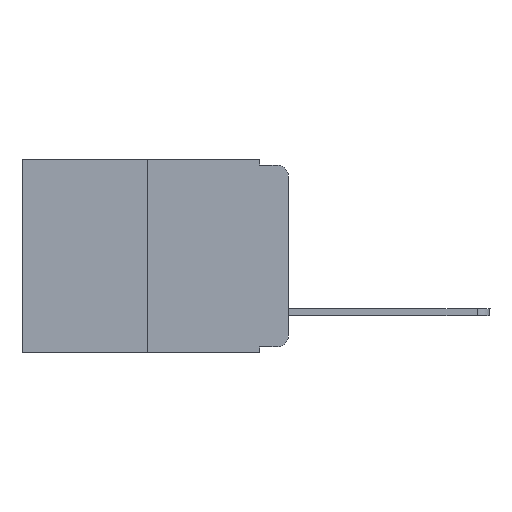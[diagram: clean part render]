
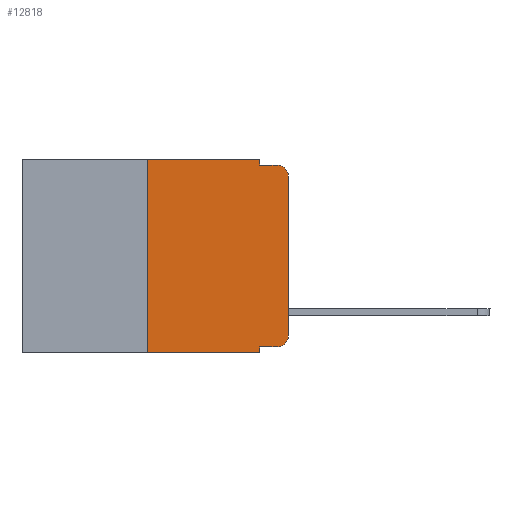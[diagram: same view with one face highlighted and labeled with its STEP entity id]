
A CAD part, left-side view. The second image highlights one B-rep face of the part: STEP entity #12818.
In plain terms, the highlighted planar face has unit normal (-1, 0, 0).
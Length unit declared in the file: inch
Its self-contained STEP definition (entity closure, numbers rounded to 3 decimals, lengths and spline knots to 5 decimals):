
#192 = EDGE_CURVE ( 'NONE', #7044, #3270, #7490, .T. ) ;
#463 = VERTEX_POINT ( 'NONE', #9555 ) ;
#1006 = LINE ( 'NONE', #9813, #6405 ) ;
#1018 = CARTESIAN_POINT ( 'NONE',  ( 0., 0.473, 0. ) ) ;
#1145 = AXIS2_PLACEMENT_3D ( 'NONE', #3611, #9482, #13429 ) ;
#1820 = DIRECTION ( 'NONE',  ( 0., 0., -1. ) ) ;
#1990 = EDGE_CURVE ( 'NONE', #8932, #7297, #15611, .T. ) ;
#1995 = PLANE ( 'NONE',  #15083 ) ;
#2068 = VERTEX_POINT ( 'NONE', #6942 ) ;
#2257 = CARTESIAN_POINT ( 'NONE',  ( 0., 0.25, -0.343 ) ) ;
#2738 = EDGE_CURVE ( 'NONE', #10157, #8932, #6647, .T. ) ;
#3189 = VECTOR ( 'NONE', #4112, 39.37008 ) ;
#3270 = VERTEX_POINT ( 'NONE', #12765 ) ;
#3534 = DIRECTION ( 'NONE',  ( 0., -1., 0. ) ) ;
#3611 = CARTESIAN_POINT ( 'NONE',  ( 0., 0.02, -0.313 ) ) ;
#3808 = DIRECTION ( 'NONE',  ( 0., -1., 0. ) ) ;
#3814 = VECTOR ( 'NONE', #12102, 39.37008 ) ;
#3880 = VECTOR ( 'NONE', #3808, 39.37008 ) ;
#3936 = LINE ( 'NONE', #11464, #10862 ) ;
#4112 = DIRECTION ( 'NONE',  ( 0., 0., -1. ) ) ;
#4262 = FACE_OUTER_BOUND ( 'NONE', #16108, .T. ) ;
#4458 = EDGE_CURVE ( 'NONE', #2068, #7297, #8194, .T. ) ;
#5738 = CARTESIAN_POINT ( 'NONE',  ( 0., 0.473, 0. ) ) ;
#6397 = EDGE_CURVE ( 'NONE', #6426, #463, #15755, .T. ) ;
#6405 = VECTOR ( 'NONE', #13422, 39.37008 ) ;
#6426 = VERTEX_POINT ( 'NONE', #2257 ) ;
#6464 = CARTESIAN_POINT ( 'NONE',  ( 0., 0.051, 0. ) ) ;
#6521 = VERTEX_POINT ( 'NONE', #15089 ) ;
#6546 = DIRECTION ( 'NONE',  ( 0., 0., 1. ) ) ;
#6647 = LINE ( 'NONE', #11637, #3189 ) ;
#6942 = CARTESIAN_POINT ( 'NONE',  ( 0., 0., -0.03 ) ) ;
#6982 = ORIENTED_EDGE ( 'NONE', *, *, #13078, .F. ) ;
#7044 = VERTEX_POINT ( 'NONE', #11394 ) ;
#7120 = CARTESIAN_POINT ( 'NONE',  ( 0., 0.25, 0. ) ) ;
#7176 = DIRECTION ( 'NONE',  ( 0., -1., 0. ) ) ;
#7294 = LINE ( 'NONE', #1018, #14986 ) ;
#7297 = VERTEX_POINT ( 'NONE', #8346 ) ;
#7319 = EDGE_CURVE ( 'NONE', #3270, #11109, #9739, .T. ) ;
#7322 = CARTESIAN_POINT ( 'NONE',  ( 0., 0.473, -0.343 ) ) ;
#7490 = LINE ( 'NONE', #10009, #3880 ) ;
#7603 = VECTOR ( 'NONE', #7176, 39.37008 ) ;
#7638 = ORIENTED_EDGE ( 'NONE', *, *, #4458, .T. ) ;
#7950 = DIRECTION ( 'NONE',  ( 1., 0., 0. ) ) ;
#8143 = ORIENTED_EDGE ( 'NONE', *, *, #14740, .F. ) ;
#8194 = CIRCLE ( 'NONE', #10285, 0.02 ) ;
#8345 = ORIENTED_EDGE ( 'NONE', *, *, #14412, .T. ) ;
#8346 = CARTESIAN_POINT ( 'NONE',  ( 0., 0.02, -0.01 ) ) ;
#8415 = LINE ( 'NONE', #7120, #3814 ) ;
#8932 = VERTEX_POINT ( 'NONE', #11585 ) ;
#9482 = DIRECTION ( 'NONE',  ( -1., 0., 0. ) ) ;
#9555 = CARTESIAN_POINT ( 'NONE',  ( 0., 0.051, -0.343 ) ) ;
#9639 = ORIENTED_EDGE ( 'NONE', *, *, #7319, .T. ) ;
#9739 = CIRCLE ( 'NONE', #1145, 0.02 ) ;
#9743 = ORIENTED_EDGE ( 'NONE', *, *, #16048, .F. ) ;
#9813 = CARTESIAN_POINT ( 'NONE',  ( 0., 0.051, 0. ) ) ;
#10009 = CARTESIAN_POINT ( 'NONE',  ( 0., 0.051, -0.333 ) ) ;
#10157 = VERTEX_POINT ( 'NONE', #6464 ) ;
#10285 = AXIS2_PLACEMENT_3D ( 'NONE', #13583, #12343, #16124 ) ;
#10467 = ORIENTED_EDGE ( 'NONE', *, *, #192, .T. ) ;
#10533 = CARTESIAN_POINT ( 'NONE',  ( 0., 0.051, -0.01 ) ) ;
#10851 = ORIENTED_EDGE ( 'NONE', *, *, #6397, .T. ) ;
#10862 = VECTOR ( 'NONE', #6546, 39.37008 ) ;
#11093 = DIRECTION ( 'NONE',  ( 0., -1., 0. ) ) ;
#11109 = VERTEX_POINT ( 'NONE', #14093 ) ;
#11394 = CARTESIAN_POINT ( 'NONE',  ( 0., 0.051, -0.333 ) ) ;
#11464 = CARTESIAN_POINT ( 'NONE',  ( 0., 0., 0. ) ) ;
#11585 = CARTESIAN_POINT ( 'NONE',  ( 0., 0.051, -0.01 ) ) ;
#11637 = CARTESIAN_POINT ( 'NONE',  ( 0., 0.051, 0. ) ) ;
#12102 = DIRECTION ( 'NONE',  ( 0., 0., 1. ) ) ;
#12343 = DIRECTION ( 'NONE',  ( -1., 0., 0. ) ) ;
#12765 = CARTESIAN_POINT ( 'NONE',  ( 0., 0.02, -0.333 ) ) ;
#12818 = ADVANCED_FACE ( 'NONE', ( #4262 ), #1995, .F. ) ;
#12861 = ORIENTED_EDGE ( 'NONE', *, *, #2738, .F. ) ;
#12961 = VECTOR ( 'NONE', #11093, 39.37008 ) ;
#13078 = EDGE_CURVE ( 'NONE', #6521, #10157, #7294, .T. ) ;
#13096 = ORIENTED_EDGE ( 'NONE', *, *, #1990, .F. ) ;
#13422 = DIRECTION ( 'NONE',  ( 0., 0., -1. ) ) ;
#13429 = DIRECTION ( 'NONE',  ( 0., 0., -1. ) ) ;
#13583 = CARTESIAN_POINT ( 'NONE',  ( 0., 0.02, -0.03 ) ) ;
#14093 = CARTESIAN_POINT ( 'NONE',  ( 0., 0., -0.313 ) ) ;
#14412 = EDGE_CURVE ( 'NONE', #11109, #2068, #3936, .T. ) ;
#14740 = EDGE_CURVE ( 'NONE', #6426, #6521, #8415, .T. ) ;
#14986 = VECTOR ( 'NONE', #3534, 39.37008 ) ;
#15083 = AXIS2_PLACEMENT_3D ( 'NONE', #5738, #7950, #1820 ) ;
#15089 = CARTESIAN_POINT ( 'NONE',  ( 0., 0.25, 0. ) ) ;
#15611 = LINE ( 'NONE', #10533, #7603 ) ;
#15755 = LINE ( 'NONE', #7322, #12961 ) ;
#16048 = EDGE_CURVE ( 'NONE', #7044, #463, #1006, .T. ) ;
#16108 = EDGE_LOOP ( 'NONE', ( #8345, #7638, #13096, #12861, #6982, #8143, #10851, #9743, #10467, #9639 ) ) ;
#16124 = DIRECTION ( 'NONE',  ( 0., 0., -1. ) ) ;
